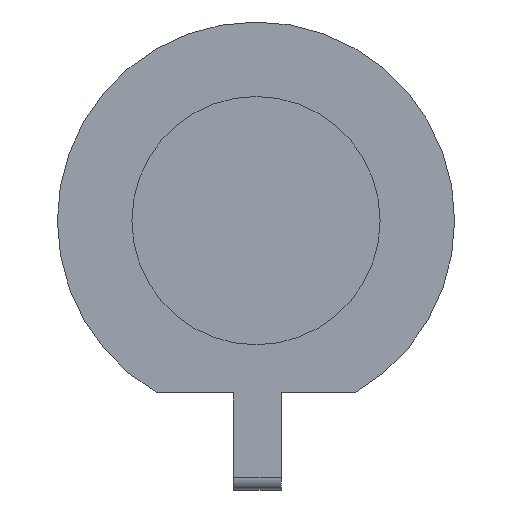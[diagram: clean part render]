
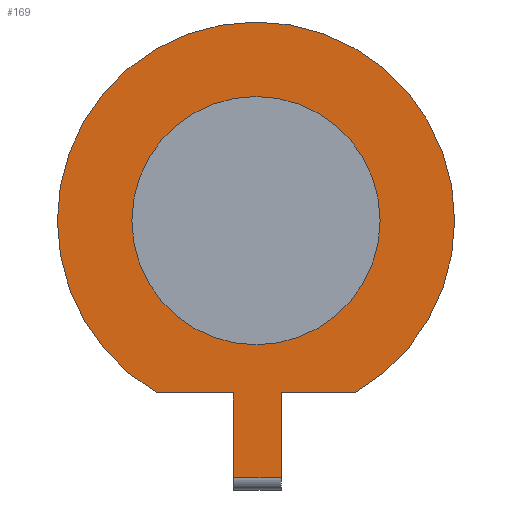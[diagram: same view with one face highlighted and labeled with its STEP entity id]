
A CAD part, front view. The second image highlights one B-rep face of the part: STEP entity #169.
In plain terms, the highlighted planar face has unit normal (0, -1, 0).
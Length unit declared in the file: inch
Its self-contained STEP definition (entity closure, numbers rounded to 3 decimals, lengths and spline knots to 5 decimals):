
#7 = VECTOR ( 'NONE', #478, 39.37008 ) ;
#22 = VERTEX_POINT ( 'NONE', #707 ) ;
#26 = DIRECTION ( 'NONE',  ( 0., 0., 1. ) ) ;
#30 = EDGE_LOOP ( 'NONE', ( #518, #455 ) ) ;
#35 = EDGE_CURVE ( 'NONE', #355, #22, #220, .T. ) ;
#42 = ORIENTED_EDGE ( 'NONE', *, *, #35, .T. ) ;
#54 = CARTESIAN_POINT ( 'NONE',  ( 0., 0., 0.5 ) ) ;
#84 = DIRECTION ( 'NONE',  ( 0., 0., 1. ) ) ;
#117 = LINE ( 'NONE', #344, #401 ) ;
#118 = VECTOR ( 'NONE', #734, 39.37008 ) ;
#120 = VERTEX_POINT ( 'NONE', #314 ) ;
#135 = EDGE_CURVE ( 'NONE', #508, #464, #642, .T. ) ;
#145 = EDGE_CURVE ( 'NONE', #282, #199, #300, .T. ) ;
#169 = ADVANCED_FACE ( 'NONE', ( #448, #564 ), #442, .F. ) ;
#185 = LINE ( 'NONE', #468, #7 ) ;
#192 = CARTESIAN_POINT ( 'NONE',  ( 0., 0., 0. ) ) ;
#199 = VERTEX_POINT ( 'NONE', #430 ) ;
#200 = CARTESIAN_POINT ( 'NONE',  ( 0.10256, 0., 0. ) ) ;
#220 = LINE ( 'NONE', #529, #363 ) ;
#221 = ORIENTED_EDGE ( 'NONE', *, *, #544, .F. ) ;
#234 = EDGE_CURVE ( 'NONE', #199, #355, #572, .T. ) ;
#244 = CARTESIAN_POINT ( 'NONE',  ( 0., 0., 0. ) ) ;
#282 = VERTEX_POINT ( 'NONE', #325 ) ;
#300 = LINE ( 'NONE', #552, #118 ) ;
#314 = CARTESIAN_POINT ( 'NONE',  ( -0.39779, 0., -0.69409 ) ) ;
#325 = CARTESIAN_POINT ( 'NONE',  ( -0.09075, 0., -1.03496 ) ) ;
#335 = CARTESIAN_POINT ( 'NONE',  ( 0.10256, 0., -0.69245 ) ) ;
#344 = CARTESIAN_POINT ( 'NONE',  ( -0.09075, 0., -0.69409 ) ) ;
#347 = CARTESIAN_POINT ( 'NONE',  ( 0., 0., -0.5 ) ) ;
#355 = VERTEX_POINT ( 'NONE', #335 ) ;
#360 = DIRECTION ( 'NONE',  ( 0., 0., -1. ) ) ;
#361 = DIRECTION ( 'NONE',  ( 0., 0., 1. ) ) ;
#363 = VECTOR ( 'NONE', #718, 39.37008 ) ;
#365 = ORIENTED_EDGE ( 'NONE', *, *, #145, .T. ) ;
#370 = CARTESIAN_POINT ( 'NONE',  ( 0., 0., 0. ) ) ;
#381 = AXIS2_PLACEMENT_3D ( 'NONE', #370, #434, #84 ) ;
#385 = VECTOR ( 'NONE', #26, 39.37008 ) ;
#401 = VECTOR ( 'NONE', #603, 39.37008 ) ;
#410 = AXIS2_PLACEMENT_3D ( 'NONE', #244, #659, #360 ) ;
#428 = CARTESIAN_POINT ( 'NONE',  ( 0., 0., 0. ) ) ;
#430 = CARTESIAN_POINT ( 'NONE',  ( 0.10256, 0., -1.03496 ) ) ;
#434 = DIRECTION ( 'NONE',  ( 0., 1., 0. ) ) ;
#440 = ORIENTED_EDGE ( 'NONE', *, *, #234, .T. ) ;
#442 = PLANE ( 'NONE',  #381 ) ;
#448 = FACE_OUTER_BOUND ( 'NONE', #768, .T. ) ;
#453 = AXIS2_PLACEMENT_3D ( 'NONE', #192, #665, #361 ) ;
#455 = ORIENTED_EDGE ( 'NONE', *, *, #135, .T. ) ;
#464 = VERTEX_POINT ( 'NONE', #347 ) ;
#468 = CARTESIAN_POINT ( 'NONE',  ( -0.09075, 0., 0. ) ) ;
#477 = ORIENTED_EDGE ( 'NONE', *, *, #560, .T. ) ;
#478 = DIRECTION ( 'NONE',  ( 0., 0., 1. ) ) ;
#480 = AXIS2_PLACEMENT_3D ( 'NONE', #428, #484, #542 ) ;
#484 = DIRECTION ( 'NONE',  ( 0., 1., 0. ) ) ;
#508 = VERTEX_POINT ( 'NONE', #54 ) ;
#518 = ORIENTED_EDGE ( 'NONE', *, *, #625, .T. ) ;
#527 = VERTEX_POINT ( 'NONE', #710 ) ;
#529 = CARTESIAN_POINT ( 'NONE',  ( 0.10256, 0., -0.69245 ) ) ;
#542 = DIRECTION ( 'NONE',  ( 0., 0., 1. ) ) ;
#544 = EDGE_CURVE ( 'NONE', #282, #527, #185, .T. ) ;
#552 = CARTESIAN_POINT ( 'NONE',  ( 0.10256, 0., -1.03496 ) ) ;
#560 = EDGE_CURVE ( 'NONE', #120, #527, #117, .T. ) ;
#564 = FACE_BOUND ( 'NONE', #30, .T. ) ;
#572 = LINE ( 'NONE', #200, #385 ) ;
#603 = DIRECTION ( 'NONE',  ( 1., 0., 0. ) ) ;
#611 = EDGE_CURVE ( 'NONE', #22, #120, #764, .T. ) ;
#625 = EDGE_CURVE ( 'NONE', #464, #508, #674, .T. ) ;
#642 = CIRCLE ( 'NONE', #453, 0.5 ) ;
#659 = DIRECTION ( 'NONE',  ( 0., -1., 0. ) ) ;
#665 = DIRECTION ( 'NONE',  ( 0., 1., 0. ) ) ;
#674 = CIRCLE ( 'NONE', #480, 0.5 ) ;
#707 = CARTESIAN_POINT ( 'NONE',  ( 0.40065, 0., -0.69245 ) ) ;
#710 = CARTESIAN_POINT ( 'NONE',  ( -0.09075, 0., -0.69409 ) ) ;
#718 = DIRECTION ( 'NONE',  ( 1., 0., 0. ) ) ;
#734 = DIRECTION ( 'NONE',  ( 1., 0., 0. ) ) ;
#748 = ORIENTED_EDGE ( 'NONE', *, *, #611, .T. ) ;
#764 = CIRCLE ( 'NONE', #410, 0.8 ) ;
#768 = EDGE_LOOP ( 'NONE', ( #477, #221, #365, #440, #42, #748 ) ) ;
